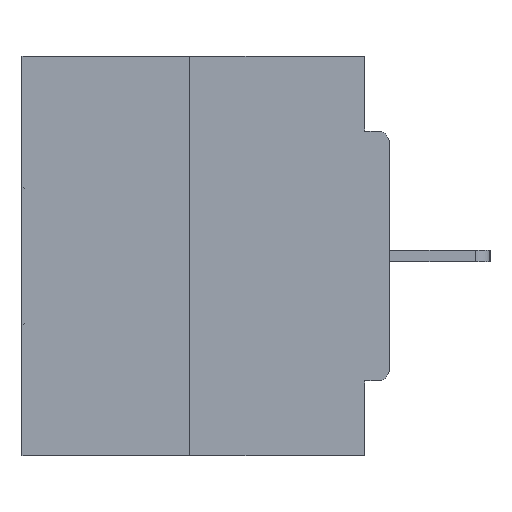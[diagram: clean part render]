
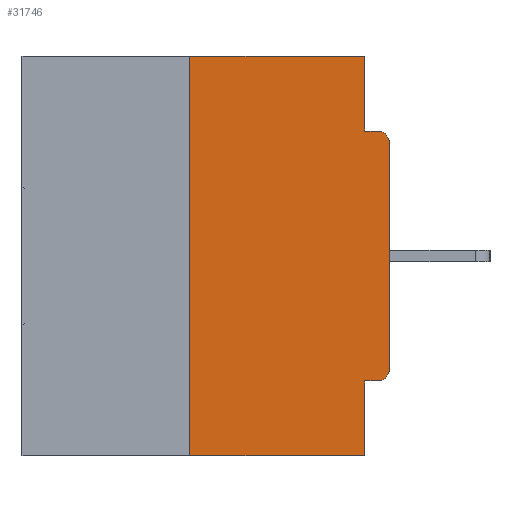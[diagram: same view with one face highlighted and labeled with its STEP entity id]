
A CAD part, left-side view. The second image highlights one B-rep face of the part: STEP entity #31746.
In plain terms, the highlighted planar face has unit normal (-1, 0, 0).
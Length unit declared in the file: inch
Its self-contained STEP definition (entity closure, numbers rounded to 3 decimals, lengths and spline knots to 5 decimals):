
#186 = VECTOR ( 'NONE', #22256, 39.37008 ) ;
#421 = ORIENTED_EDGE ( 'NONE', *, *, #14926, .F. ) ;
#489 = CARTESIAN_POINT ( 'NONE',  ( 0., 0.015, -0.0935 ) ) ;
#1099 = EDGE_CURVE ( 'NONE', #10992, #7905, #16007, .T. ) ;
#2161 = ORIENTED_EDGE ( 'NONE', *, *, #25741, .T. ) ;
#2260 = ORIENTED_EDGE ( 'NONE', *, *, #19006, .F. ) ;
#2263 = FACE_OUTER_BOUND ( 'NONE', #6749, .T. ) ;
#3196 = LINE ( 'NONE', #18525, #13333 ) ;
#3575 = VERTEX_POINT ( 'NONE', #15671 ) ;
#3603 = DIRECTION ( 'NONE',  ( 0., -1., 0. ) ) ;
#3895 = CARTESIAN_POINT ( 'NONE',  ( 0., 0.015, -0.4065 ) ) ;
#4115 = VECTOR ( 'NONE', #24623, 39.37008 ) ;
#4121 = CIRCLE ( 'NONE', #22150, 0.015 ) ;
#4572 = DIRECTION ( 'NONE',  ( 0., 0., -1. ) ) ;
#5830 = ORIENTED_EDGE ( 'NONE', *, *, #28529, .T. ) ;
#6222 = CARTESIAN_POINT ( 'NONE',  ( 0., 0.031, 0. ) ) ;
#6749 = EDGE_LOOP ( 'NONE', ( #21729, #22442, #31386, #421, #19969, #5830, #2161, #22708, #31734, #2260 ) ) ;
#7346 = DIRECTION ( 'NONE',  ( 0., 0., -1. ) ) ;
#7905 = VERTEX_POINT ( 'NONE', #31841 ) ;
#8401 = VERTEX_POINT ( 'NONE', #489 ) ;
#8446 = LINE ( 'NONE', #16393, #29183 ) ;
#9910 = DIRECTION ( 'NONE',  ( 1., 0., 0. ) ) ;
#10141 = CARTESIAN_POINT ( 'NONE',  ( 0., 0.46, 0. ) ) ;
#10729 = CIRCLE ( 'NONE', #11143, 0.015 ) ;
#10876 = LINE ( 'NONE', #19106, #4115 ) ;
#10992 = VERTEX_POINT ( 'NONE', #11931 ) ;
#10996 = DIRECTION ( 'NONE',  ( 0., 0., 1. ) ) ;
#11143 = AXIS2_PLACEMENT_3D ( 'NONE', #23530, #28854, #7346 ) ;
#11395 = VECTOR ( 'NONE', #21174, 39.37008 ) ;
#11863 = CARTESIAN_POINT ( 'NONE',  ( 0., 0.031, -0.5 ) ) ;
#11931 = CARTESIAN_POINT ( 'NONE',  ( 0., 0.25, 0. ) ) ;
#13333 = VECTOR ( 'NONE', #23804, 39.37008 ) ;
#13489 = EDGE_CURVE ( 'NONE', #18604, #19561, #21063, .T. ) ;
#13675 = CARTESIAN_POINT ( 'NONE',  ( 0., 0.031, -0.0935 ) ) ;
#13969 = EDGE_CURVE ( 'NONE', #18604, #10992, #29945, .T. ) ;
#14028 = CARTESIAN_POINT ( 'NONE',  ( 0., 0., 0. ) ) ;
#14838 = VECTOR ( 'NONE', #22413, 39.37008 ) ;
#14926 = EDGE_CURVE ( 'NONE', #34202, #19561, #10876, .T. ) ;
#15427 = LINE ( 'NONE', #14028, #186 ) ;
#15671 = CARTESIAN_POINT ( 'NONE',  ( 0., 0., -0.1085 ) ) ;
#16007 = LINE ( 'NONE', #10141, #11395 ) ;
#16393 = CARTESIAN_POINT ( 'NONE',  ( 0., 0., -0.0935 ) ) ;
#18525 = CARTESIAN_POINT ( 'NONE',  ( 0., 0., -0.4065 ) ) ;
#18604 = VERTEX_POINT ( 'NONE', #19730 ) ;
#19006 = EDGE_CURVE ( 'NONE', #7905, #30344, #22023, .T. ) ;
#19010 = DIRECTION ( 'NONE',  ( 0., -1., 0. ) ) ;
#19106 = CARTESIAN_POINT ( 'NONE',  ( 0., 0.031, -0.5 ) ) ;
#19343 = EDGE_CURVE ( 'NONE', #30344, #8401, #8446, .T. ) ;
#19561 = VERTEX_POINT ( 'NONE', #11863 ) ;
#19730 = CARTESIAN_POINT ( 'NONE',  ( 0., 0.25, -0.5 ) ) ;
#19969 = ORIENTED_EDGE ( 'NONE', *, *, #29715, .F. ) ;
#20619 = VECTOR ( 'NONE', #3603, 39.37008 ) ;
#20930 = PLANE ( 'NONE',  #35006 ) ;
#21063 = LINE ( 'NONE', #33306, #20619 ) ;
#21174 = DIRECTION ( 'NONE',  ( 0., -1., 0. ) ) ;
#21647 = CARTESIAN_POINT ( 'NONE',  ( 0., 0.25, 0. ) ) ;
#21729 = ORIENTED_EDGE ( 'NONE', *, *, #1099, .F. ) ;
#22023 = LINE ( 'NONE', #6222, #14838 ) ;
#22150 = AXIS2_PLACEMENT_3D ( 'NONE', #28837, #28721, #31449 ) ;
#22256 = DIRECTION ( 'NONE',  ( 0., 0., 1. ) ) ;
#22413 = DIRECTION ( 'NONE',  ( 0., 0., -1. ) ) ;
#22442 = ORIENTED_EDGE ( 'NONE', *, *, #13969, .F. ) ;
#22708 = ORIENTED_EDGE ( 'NONE', *, *, #31221, .T. ) ;
#22742 = VECTOR ( 'NONE', #10996, 39.37008 ) ;
#23530 = CARTESIAN_POINT ( 'NONE',  ( 0., 0.015, -0.1085 ) ) ;
#23804 = DIRECTION ( 'NONE',  ( 0., 1., 0. ) ) ;
#24623 = DIRECTION ( 'NONE',  ( 0., 0., -1. ) ) ;
#25741 = EDGE_CURVE ( 'NONE', #34881, #3575, #15427, .T. ) ;
#26357 = VERTEX_POINT ( 'NONE', #3895 ) ;
#28529 = EDGE_CURVE ( 'NONE', #26357, #34881, #4121, .T. ) ;
#28721 = DIRECTION ( 'NONE',  ( -1., 0., 0. ) ) ;
#28837 = CARTESIAN_POINT ( 'NONE',  ( 0., 0.015, -0.3915 ) ) ;
#28854 = DIRECTION ( 'NONE',  ( -1., 0., 0. ) ) ;
#29183 = VECTOR ( 'NONE', #19010, 39.37008 ) ;
#29384 = CARTESIAN_POINT ( 'NONE',  ( 0., 0.031, -0.4065 ) ) ;
#29715 = EDGE_CURVE ( 'NONE', #26357, #34202, #3196, .T. ) ;
#29945 = LINE ( 'NONE', #21647, #22742 ) ;
#30133 = CARTESIAN_POINT ( 'NONE',  ( 0., 0., -0.3915 ) ) ;
#30344 = VERTEX_POINT ( 'NONE', #13675 ) ;
#31221 = EDGE_CURVE ( 'NONE', #3575, #8401, #10729, .T. ) ;
#31386 = ORIENTED_EDGE ( 'NONE', *, *, #13489, .T. ) ;
#31449 = DIRECTION ( 'NONE',  ( 0., 0., -1. ) ) ;
#31671 = CARTESIAN_POINT ( 'NONE',  ( 0., 0.46, 0. ) ) ;
#31734 = ORIENTED_EDGE ( 'NONE', *, *, #19343, .F. ) ;
#31746 = ADVANCED_FACE ( 'NONE', ( #2263 ), #20930, .F. ) ;
#31841 = CARTESIAN_POINT ( 'NONE',  ( 0., 0.031, 0. ) ) ;
#33306 = CARTESIAN_POINT ( 'NONE',  ( 0., 0.46, -0.5 ) ) ;
#34202 = VERTEX_POINT ( 'NONE', #29384 ) ;
#34881 = VERTEX_POINT ( 'NONE', #30133 ) ;
#35006 = AXIS2_PLACEMENT_3D ( 'NONE', #31671, #9910, #4572 ) ;
